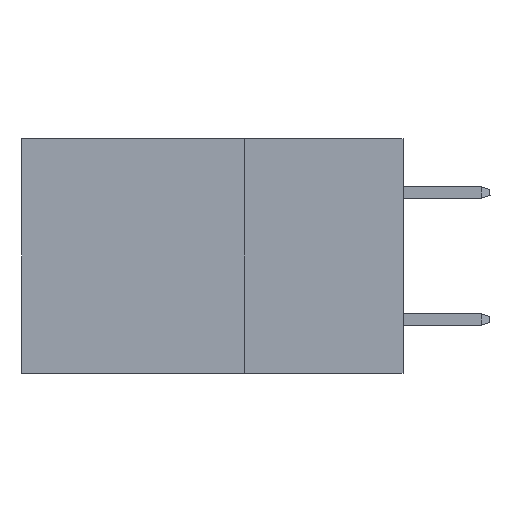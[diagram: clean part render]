
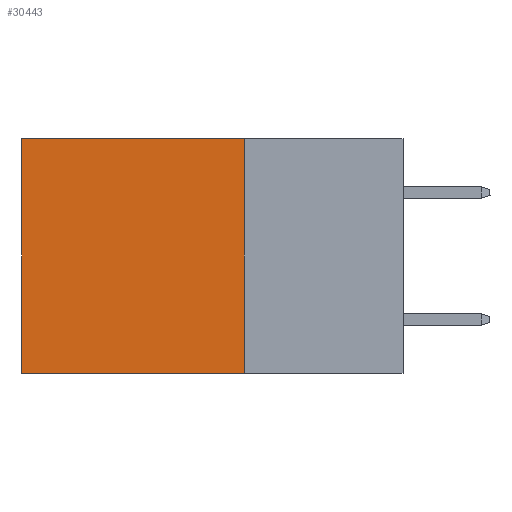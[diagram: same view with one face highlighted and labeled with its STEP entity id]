
A CAD part, left-side view. The second image highlights one B-rep face of the part: STEP entity #30443.
In plain terms, the highlighted planar face has unit normal (-1, 0, 0).
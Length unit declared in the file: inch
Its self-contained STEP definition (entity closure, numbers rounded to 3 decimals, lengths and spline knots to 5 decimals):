
#169 = DIRECTION ( 'NONE',  ( 0., 1., 0. ) ) ;
#1770 = LINE ( 'NONE', #28740, #14830 ) ;
#4428 = EDGE_LOOP ( 'NONE', ( #7335, #9775, #39721, #22201 ) ) ;
#4650 = DIRECTION ( 'NONE',  ( 1., 0., 0. ) ) ;
#6801 = VERTEX_POINT ( 'NONE', #7099 ) ;
#7099 = CARTESIAN_POINT ( 'NONE',  ( 0.2875, 0.6, 0. ) ) ;
#7335 = ORIENTED_EDGE ( 'NONE', *, *, #37842, .T. ) ;
#8381 = VERTEX_POINT ( 'NONE', #9901 ) ;
#8497 = CARTESIAN_POINT ( 'NONE',  ( 0.2875, 0.6, 0. ) ) ;
#9775 = ORIENTED_EDGE ( 'NONE', *, *, #17829, .F. ) ;
#9901 = CARTESIAN_POINT ( 'NONE',  ( 0.2875, 0.6, -0.37 ) ) ;
#10481 = CARTESIAN_POINT ( 'NONE',  ( 0.2875, 0.25, -0.37 ) ) ;
#11851 = DIRECTION ( 'NONE',  ( 0., 0., -1. ) ) ;
#12641 = LINE ( 'NONE', #19737, #15484 ) ;
#13482 = VECTOR ( 'NONE', #11851, 39.37008 ) ;
#14830 = VECTOR ( 'NONE', #18471, 39.37008 ) ;
#15334 = FACE_OUTER_BOUND ( 'NONE', #4428, .T. ) ;
#15484 = VECTOR ( 'NONE', #16393, 39.37008 ) ;
#16393 = DIRECTION ( 'NONE',  ( 0., 0., -1. ) ) ;
#16681 = LINE ( 'NONE', #10481, #34896 ) ;
#17829 = EDGE_CURVE ( 'NONE', #24917, #8381, #16681, .T. ) ;
#18471 = DIRECTION ( 'NONE',  ( 0., 1., 0. ) ) ;
#19737 = CARTESIAN_POINT ( 'NONE',  ( 0.2875, 0.25, 0. ) ) ;
#20221 = VERTEX_POINT ( 'NONE', #41742 ) ;
#22201 = ORIENTED_EDGE ( 'NONE', *, *, #33689, .T. ) ;
#24917 = VERTEX_POINT ( 'NONE', #32785 ) ;
#25361 = DIRECTION ( 'NONE',  ( 0., 0., -1. ) ) ;
#25575 = PLANE ( 'NONE',  #40092 ) ;
#28740 = CARTESIAN_POINT ( 'NONE',  ( 0.2875, 0.25, 0. ) ) ;
#28769 = LINE ( 'NONE', #8497, #13482 ) ;
#30443 = ADVANCED_FACE ( 'NONE', ( #15334 ), #25575, .F. ) ;
#32785 = CARTESIAN_POINT ( 'NONE',  ( 0.2875, 0.25, -0.37 ) ) ;
#33689 = EDGE_CURVE ( 'NONE', #20221, #6801, #1770, .T. ) ;
#34896 = VECTOR ( 'NONE', #169, 39.37008 ) ;
#35477 = EDGE_CURVE ( 'NONE', #20221, #24917, #12641, .T. ) ;
#37842 = EDGE_CURVE ( 'NONE', #6801, #8381, #28769, .T. ) ;
#39105 = CARTESIAN_POINT ( 'NONE',  ( 0.2875, 0.25, 0. ) ) ;
#39721 = ORIENTED_EDGE ( 'NONE', *, *, #35477, .F. ) ;
#40092 = AXIS2_PLACEMENT_3D ( 'NONE', #39105, #4650, #25361 ) ;
#41742 = CARTESIAN_POINT ( 'NONE',  ( 0.2875, 0.25, 0. ) ) ;
